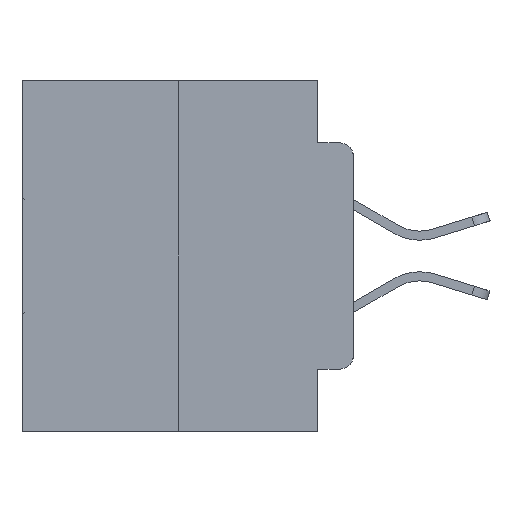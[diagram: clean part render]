
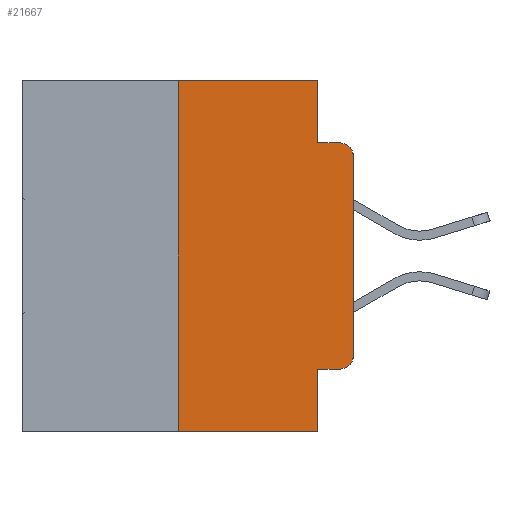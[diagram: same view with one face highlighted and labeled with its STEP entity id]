
A CAD part, left-side view. The second image highlights one B-rep face of the part: STEP entity #21667.
In plain terms, the highlighted planar face has unit normal (-1, 0, 0).
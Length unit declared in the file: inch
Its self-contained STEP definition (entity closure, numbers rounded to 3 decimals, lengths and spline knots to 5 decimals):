
#146 = DIRECTION ( 'NONE',  ( 0., 0., 1. ) ) ;
#486 = EDGE_CURVE ( 'NONE', #22147, #1114, #5234, .T. ) ;
#544 = ORIENTED_EDGE ( 'NONE', *, *, #22656, .T. ) ;
#588 = CIRCLE ( 'NONE', #17471, 0.02 ) ;
#636 = CARTESIAN_POINT ( 'NONE',  ( 0., 0.051, 0. ) ) ;
#799 = VECTOR ( 'NONE', #146, 39.37008 ) ;
#909 = ORIENTED_EDGE ( 'NONE', *, *, #13636, .F. ) ;
#1040 = VERTEX_POINT ( 'NONE', #20191 ) ;
#1114 = VERTEX_POINT ( 'NONE', #10841 ) ;
#1234 = CARTESIAN_POINT ( 'NONE',  ( 0., 0.051, -0.5 ) ) ;
#1327 = EDGE_CURVE ( 'NONE', #1040, #11623, #588, .T. ) ;
#1612 = DIRECTION ( 'NONE',  ( 0., 0., -1. ) ) ;
#1700 = VECTOR ( 'NONE', #7010, 39.37008 ) ;
#1853 = CARTESIAN_POINT ( 'NONE',  ( 0., 0.051, -0.4115 ) ) ;
#2376 = EDGE_LOOP ( 'NONE', ( #544, #11352, #20029, #26877, #909, #10388, #28555, #9665, #17860, #26222 ) ) ;
#2642 = EDGE_CURVE ( 'NONE', #17299, #5890, #7620, .T. ) ;
#3474 = CARTESIAN_POINT ( 'NONE',  ( 0., 0.02, -0.1085 ) ) ;
#4473 = VERTEX_POINT ( 'NONE', #16786 ) ;
#4834 = CARTESIAN_POINT ( 'NONE',  ( 0., 0.25, 0. ) ) ;
#5234 = CIRCLE ( 'NONE', #22110, 0.02 ) ;
#5321 = CARTESIAN_POINT ( 'NONE',  ( 0., 0.051, -0.0885 ) ) ;
#5326 = CARTESIAN_POINT ( 'NONE',  ( 0., 0., -0.3915 ) ) ;
#5890 = VERTEX_POINT ( 'NONE', #1234 ) ;
#5952 = CARTESIAN_POINT ( 'NONE',  ( 0., 0.051, 0. ) ) ;
#6006 = EDGE_CURVE ( 'NONE', #21267, #4473, #27301, .T. ) ;
#7010 = DIRECTION ( 'NONE',  ( 0., -1., 0. ) ) ;
#7501 = DIRECTION ( 'NONE',  ( 1., 0., 0. ) ) ;
#7620 = LINE ( 'NONE', #5952, #9440 ) ;
#7766 = VERTEX_POINT ( 'NONE', #12811 ) ;
#7990 = CARTESIAN_POINT ( 'NONE',  ( 0., 0., 0. ) ) ;
#8420 = CARTESIAN_POINT ( 'NONE',  ( 0., 0.473, 0. ) ) ;
#8470 = CARTESIAN_POINT ( 'NONE',  ( 0., 0., -0.1085 ) ) ;
#9440 = VECTOR ( 'NONE', #17141, 39.37008 ) ;
#9665 = ORIENTED_EDGE ( 'NONE', *, *, #2642, .F. ) ;
#9788 = PLANE ( 'NONE',  #10725 ) ;
#9866 = VECTOR ( 'NONE', #29207, 39.37008 ) ;
#10199 = EDGE_CURVE ( 'NONE', #7766, #1114, #11678, .T. ) ;
#10388 = ORIENTED_EDGE ( 'NONE', *, *, #6006, .F. ) ;
#10725 = AXIS2_PLACEMENT_3D ( 'NONE', #18992, #7501, #25915 ) ;
#10841 = CARTESIAN_POINT ( 'NONE',  ( 0., 0.02, -0.0885 ) ) ;
#11352 = ORIENTED_EDGE ( 'NONE', *, *, #486, .T. ) ;
#11623 = VERTEX_POINT ( 'NONE', #5326 ) ;
#11678 = LINE ( 'NONE', #5321, #19584 ) ;
#12811 = CARTESIAN_POINT ( 'NONE',  ( 0., 0.051, -0.0885 ) ) ;
#13379 = LINE ( 'NONE', #15497, #9866 ) ;
#13636 = EDGE_CURVE ( 'NONE', #4473, #21979, #26978, .T. ) ;
#15462 = EDGE_CURVE ( 'NONE', #21979, #7766, #20333, .T. ) ;
#15497 = CARTESIAN_POINT ( 'NONE',  ( 0., 0.473, -0.5 ) ) ;
#15666 = DIRECTION ( 'NONE',  ( 0., -1., 0. ) ) ;
#15938 = LINE ( 'NONE', #23179, #1700 ) ;
#16163 = CARTESIAN_POINT ( 'NONE',  ( 0., 0.25, -0.5 ) ) ;
#16786 = CARTESIAN_POINT ( 'NONE',  ( 0., 0.25, 0. ) ) ;
#17141 = DIRECTION ( 'NONE',  ( 0., 0., -1. ) ) ;
#17299 = VERTEX_POINT ( 'NONE', #1853 ) ;
#17471 = AXIS2_PLACEMENT_3D ( 'NONE', #23930, #26175, #28732 ) ;
#17860 = ORIENTED_EDGE ( 'NONE', *, *, #24709, .T. ) ;
#18843 = FACE_OUTER_BOUND ( 'NONE', #2376, .T. ) ;
#18992 = CARTESIAN_POINT ( 'NONE',  ( 0., 0.473, 0. ) ) ;
#19174 = DIRECTION ( 'NONE',  ( 0., 0., -1. ) ) ;
#19584 = VECTOR ( 'NONE', #25551, 39.37008 ) ;
#19626 = DIRECTION ( 'NONE',  ( 0., 0., 1. ) ) ;
#20029 = ORIENTED_EDGE ( 'NONE', *, *, #10199, .F. ) ;
#20191 = CARTESIAN_POINT ( 'NONE',  ( 0., 0.02, -0.4115 ) ) ;
#20333 = LINE ( 'NONE', #28906, #21717 ) ;
#21267 = VERTEX_POINT ( 'NONE', #16163 ) ;
#21667 = ADVANCED_FACE ( 'NONE', ( #18843 ), #9788, .F. ) ;
#21717 = VECTOR ( 'NONE', #1612, 39.37008 ) ;
#21979 = VERTEX_POINT ( 'NONE', #636 ) ;
#22110 = AXIS2_PLACEMENT_3D ( 'NONE', #3474, #28799, #19174 ) ;
#22147 = VERTEX_POINT ( 'NONE', #8470 ) ;
#22656 = EDGE_CURVE ( 'NONE', #11623, #22147, #28652, .T. ) ;
#23179 = CARTESIAN_POINT ( 'NONE',  ( 0., 0.051, -0.4115 ) ) ;
#23930 = CARTESIAN_POINT ( 'NONE',  ( 0., 0.02, -0.3915 ) ) ;
#24708 = VECTOR ( 'NONE', #19626, 39.37008 ) ;
#24709 = EDGE_CURVE ( 'NONE', #17299, #1040, #15938, .T. ) ;
#25551 = DIRECTION ( 'NONE',  ( 0., -1., 0. ) ) ;
#25915 = DIRECTION ( 'NONE',  ( 0., 0., -1. ) ) ;
#25986 = EDGE_CURVE ( 'NONE', #21267, #5890, #13379, .T. ) ;
#25999 = VECTOR ( 'NONE', #15666, 39.37008 ) ;
#26175 = DIRECTION ( 'NONE',  ( -1., 0., 0. ) ) ;
#26222 = ORIENTED_EDGE ( 'NONE', *, *, #1327, .T. ) ;
#26877 = ORIENTED_EDGE ( 'NONE', *, *, #15462, .F. ) ;
#26978 = LINE ( 'NONE', #8420, #25999 ) ;
#27301 = LINE ( 'NONE', #4834, #799 ) ;
#28555 = ORIENTED_EDGE ( 'NONE', *, *, #25986, .T. ) ;
#28652 = LINE ( 'NONE', #7990, #24708 ) ;
#28732 = DIRECTION ( 'NONE',  ( 0., 0., -1. ) ) ;
#28799 = DIRECTION ( 'NONE',  ( -1., 0., 0. ) ) ;
#28906 = CARTESIAN_POINT ( 'NONE',  ( 0., 0.051, 0. ) ) ;
#29207 = DIRECTION ( 'NONE',  ( 0., -1., 0. ) ) ;
